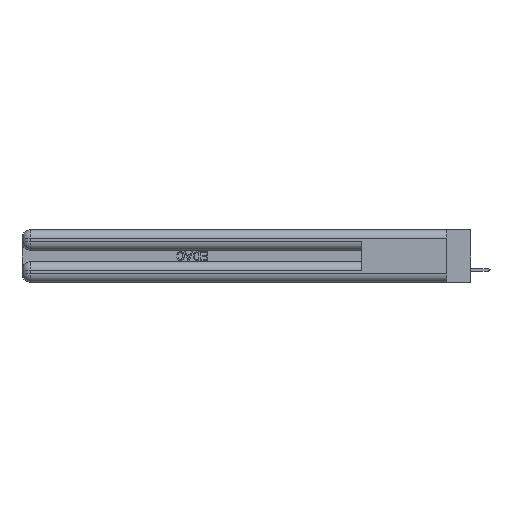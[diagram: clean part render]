
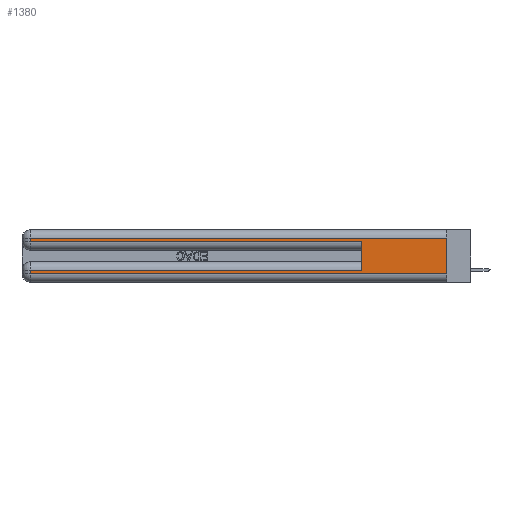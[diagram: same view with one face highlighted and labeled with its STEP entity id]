
A CAD part, left-side view. The second image highlights one B-rep face of the part: STEP entity #1380.
In plain terms, the highlighted planar face has unit normal (-1, 0, 0).
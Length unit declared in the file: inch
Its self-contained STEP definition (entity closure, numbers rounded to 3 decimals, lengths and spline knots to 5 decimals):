
#487 = EDGE_CURVE ( 'NONE', #19127, #48138, #49689, .T. ) ;
#732 = PLANE ( 'NONE',  #25000 ) ;
#1380 = ADVANCED_FACE ( 'NONE', ( #8757 ), #732, .F. ) ;
#1465 = EDGE_CURVE ( 'NONE', #36688, #34055, #42559, .T. ) ;
#1550 = CARTESIAN_POINT ( 'NONE',  ( 0., 0.6, 0.145 ) ) ;
#2006 = CARTESIAN_POINT ( 'NONE',  ( 0., 0., 0.31 ) ) ;
#2011 = EDGE_CURVE ( 'NONE', #36688, #48138, #21933, .T. ) ;
#3125 = VERTEX_POINT ( 'NONE', #46250 ) ;
#4144 = VECTOR ( 'NONE', #36729, 39.37008 ) ;
#5033 = DIRECTION ( 'NONE',  ( 0., 0., -1. ) ) ;
#5828 = DIRECTION ( 'NONE',  ( 0., 0., 1. ) ) ;
#6467 = VECTOR ( 'NONE', #29099, 39.37008 ) ;
#6586 = EDGE_LOOP ( 'NONE', ( #32190, #47651, #43982, #12220, #44539, #46353, #47605, #10183 ) ) ;
#7194 = DIRECTION ( 'NONE',  ( 0., -1., 0. ) ) ;
#8503 = EDGE_CURVE ( 'NONE', #3125, #15594, #39609, .T. ) ;
#8757 = FACE_OUTER_BOUND ( 'NONE', #6586, .T. ) ;
#9237 = DIRECTION ( 'NONE',  ( 0., 0., -1. ) ) ;
#10183 = ORIENTED_EDGE ( 'NONE', *, *, #8503, .T. ) ;
#12220 = ORIENTED_EDGE ( 'NONE', *, *, #487, .T. ) ;
#12647 = CARTESIAN_POINT ( 'NONE',  ( 0., 0., 0.285 ) ) ;
#13783 = LINE ( 'NONE', #2006, #33984 ) ;
#14326 = DIRECTION ( 'NONE',  ( 0., 1., 0. ) ) ;
#15594 = VERTEX_POINT ( 'NONE', #38434 ) ;
#17106 = CARTESIAN_POINT ( 'NONE',  ( 0., 0., 0.37 ) ) ;
#17234 = VECTOR ( 'NONE', #9237, 39.37008 ) ;
#19127 = VERTEX_POINT ( 'NONE', #25576 ) ;
#21933 = LINE ( 'NONE', #1550, #25882 ) ;
#25000 = AXIS2_PLACEMENT_3D ( 'NONE', #17106, #33415, #5033 ) ;
#25082 = LINE ( 'NONE', #25618, #17234 ) ;
#25380 = CARTESIAN_POINT ( 'NONE',  ( 0., 0., 0.31 ) ) ;
#25576 = CARTESIAN_POINT ( 'NONE',  ( 0., 2.94, 0.285 ) ) ;
#25618 = CARTESIAN_POINT ( 'NONE',  ( 0., 0., 0.37 ) ) ;
#25882 = VECTOR ( 'NONE', #5828, 39.37008 ) ;
#27492 = VECTOR ( 'NONE', #29263, 39.37008 ) ;
#28702 = LINE ( 'NONE', #45098, #4144 ) ;
#28759 = CARTESIAN_POINT ( 'NONE',  ( 0., 2.94, 0.085 ) ) ;
#29099 = DIRECTION ( 'NONE',  ( 0., 0., -1. ) ) ;
#29263 = DIRECTION ( 'NONE',  ( 0., -1., 0. ) ) ;
#31157 = EDGE_CURVE ( 'NONE', #49861, #15594, #25082, .T. ) ;
#32172 = CARTESIAN_POINT ( 'NONE',  ( 0., 0.6, 0.285 ) ) ;
#32190 = ORIENTED_EDGE ( 'NONE', *, *, #31157, .F. ) ;
#32377 = VECTOR ( 'NONE', #7194, 39.37008 ) ;
#33415 = DIRECTION ( 'NONE',  ( 1., 0., 0. ) ) ;
#33903 = LINE ( 'NONE', #50325, #6467 ) ;
#33984 = VECTOR ( 'NONE', #14326, 39.37008 ) ;
#34055 = VERTEX_POINT ( 'NONE', #28759 ) ;
#35101 = VERTEX_POINT ( 'NONE', #48897 ) ;
#35228 = VECTOR ( 'NONE', #50909, 39.37008 ) ;
#36688 = VERTEX_POINT ( 'NONE', #39984 ) ;
#36729 = DIRECTION ( 'NONE',  ( 0., 0., -1. ) ) ;
#38434 = CARTESIAN_POINT ( 'NONE',  ( 0., 0., 0.06 ) ) ;
#38502 = CARTESIAN_POINT ( 'NONE',  ( 0., 0., 0.085 ) ) ;
#39609 = LINE ( 'NONE', #52838, #32377 ) ;
#39984 = CARTESIAN_POINT ( 'NONE',  ( 0., 0.6, 0.085 ) ) ;
#41364 = EDGE_CURVE ( 'NONE', #49861, #35101, #13783, .T. ) ;
#42559 = LINE ( 'NONE', #38502, #35228 ) ;
#43982 = ORIENTED_EDGE ( 'NONE', *, *, #48713, .T. ) ;
#44539 = ORIENTED_EDGE ( 'NONE', *, *, #2011, .F. ) ;
#45098 = CARTESIAN_POINT ( 'NONE',  ( 0., 2.94, 0.37 ) ) ;
#46250 = CARTESIAN_POINT ( 'NONE',  ( 0., 2.94, 0.06 ) ) ;
#46353 = ORIENTED_EDGE ( 'NONE', *, *, #1465, .T. ) ;
#47605 = ORIENTED_EDGE ( 'NONE', *, *, #51771, .T. ) ;
#47651 = ORIENTED_EDGE ( 'NONE', *, *, #41364, .T. ) ;
#48138 = VERTEX_POINT ( 'NONE', #32172 ) ;
#48713 = EDGE_CURVE ( 'NONE', #35101, #19127, #33903, .T. ) ;
#48897 = CARTESIAN_POINT ( 'NONE',  ( 0., 2.94, 0.31 ) ) ;
#49689 = LINE ( 'NONE', #12647, #27492 ) ;
#49861 = VERTEX_POINT ( 'NONE', #25380 ) ;
#50325 = CARTESIAN_POINT ( 'NONE',  ( 0., 2.94, 0.37 ) ) ;
#50909 = DIRECTION ( 'NONE',  ( 0., 1., 0. ) ) ;
#51771 = EDGE_CURVE ( 'NONE', #34055, #3125, #28702, .T. ) ;
#52838 = CARTESIAN_POINT ( 'NONE',  ( 0., 0., 0.06 ) ) ;
